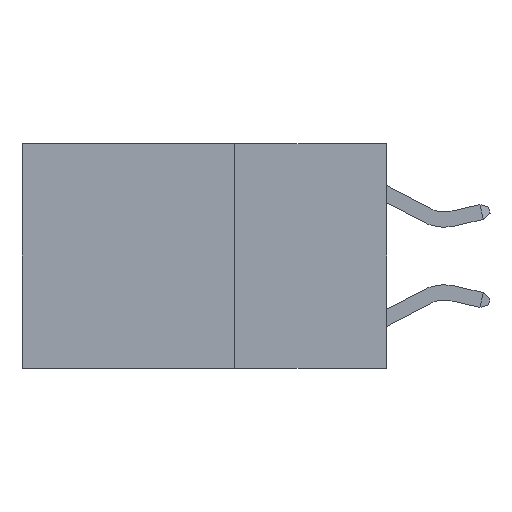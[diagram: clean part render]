
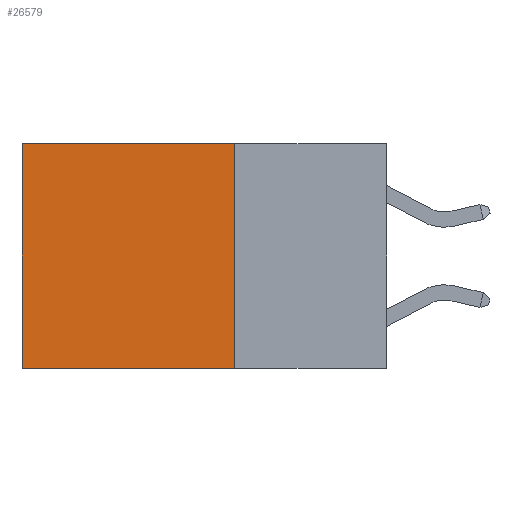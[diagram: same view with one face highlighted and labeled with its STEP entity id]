
A CAD part, left-side view. The second image highlights one B-rep face of the part: STEP entity #26579.
In plain terms, the highlighted planar face has unit normal (-1, 0, 0).
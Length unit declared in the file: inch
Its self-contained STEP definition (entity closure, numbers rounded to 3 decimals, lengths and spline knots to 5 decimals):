
#484 = CARTESIAN_POINT ( 'NONE',  ( 0.2625, 0.6, 0. ) ) ;
#586 = DIRECTION ( 'NONE',  ( 0., 0., -1. ) ) ;
#959 = EDGE_CURVE ( 'NONE', #15453, #30490, #2435, .T. ) ;
#2211 = EDGE_CURVE ( 'NONE', #25527, #30490, #9482, .T. ) ;
#2247 = VECTOR ( 'NONE', #18877, 39.37008 ) ;
#2435 = LINE ( 'NONE', #15923, #2247 ) ;
#2756 = FACE_OUTER_BOUND ( 'NONE', #12522, .T. ) ;
#3754 = CARTESIAN_POINT ( 'NONE',  ( 0.2625, 0.25, 0. ) ) ;
#5227 = CARTESIAN_POINT ( 'NONE',  ( 0.2625, 0.25, 0. ) ) ;
#5386 = ORIENTED_EDGE ( 'NONE', *, *, #21497, .F. ) ;
#6149 = VECTOR ( 'NONE', #12272, 39.37008 ) ;
#6588 = CARTESIAN_POINT ( 'NONE',  ( 0.2625, 0.6, 0. ) ) ;
#6665 = VERTEX_POINT ( 'NONE', #3754 ) ;
#9284 = EDGE_CURVE ( 'NONE', #6665, #25527, #29459, .T. ) ;
#9482 = LINE ( 'NONE', #484, #6149 ) ;
#10420 = VECTOR ( 'NONE', #10786, 39.37008 ) ;
#10786 = DIRECTION ( 'NONE',  ( 0., 1., 0. ) ) ;
#11439 = ORIENTED_EDGE ( 'NONE', *, *, #959, .F. ) ;
#12272 = DIRECTION ( 'NONE',  ( 0., 0., -1. ) ) ;
#12522 = EDGE_LOOP ( 'NONE', ( #25653, #11439, #5386, #27487 ) ) ;
#14356 = CARTESIAN_POINT ( 'NONE',  ( 0.2625, 0.25, 0. ) ) ;
#14821 = LINE ( 'NONE', #14356, #27913 ) ;
#15453 = VERTEX_POINT ( 'NONE', #19519 ) ;
#15923 = CARTESIAN_POINT ( 'NONE',  ( 0.2625, 0.25, -0.37 ) ) ;
#17041 = PLANE ( 'NONE',  #22439 ) ;
#17638 = CARTESIAN_POINT ( 'NONE',  ( 0.2625, 0.25, 0. ) ) ;
#18877 = DIRECTION ( 'NONE',  ( 0., 1., 0. ) ) ;
#19519 = CARTESIAN_POINT ( 'NONE',  ( 0.2625, 0.25, -0.37 ) ) ;
#21497 = EDGE_CURVE ( 'NONE', #6665, #15453, #14821, .T. ) ;
#22439 = AXIS2_PLACEMENT_3D ( 'NONE', #5227, #24196, #586 ) ;
#23253 = DIRECTION ( 'NONE',  ( 0., 0., -1. ) ) ;
#24196 = DIRECTION ( 'NONE',  ( 1., 0., 0. ) ) ;
#25527 = VERTEX_POINT ( 'NONE', #6588 ) ;
#25653 = ORIENTED_EDGE ( 'NONE', *, *, #2211, .T. ) ;
#26579 = ADVANCED_FACE ( 'NONE', ( #2756 ), #17041, .F. ) ;
#27487 = ORIENTED_EDGE ( 'NONE', *, *, #9284, .T. ) ;
#27654 = CARTESIAN_POINT ( 'NONE',  ( 0.2625, 0.6, -0.37 ) ) ;
#27913 = VECTOR ( 'NONE', #23253, 39.37008 ) ;
#29459 = LINE ( 'NONE', #17638, #10420 ) ;
#30490 = VERTEX_POINT ( 'NONE', #27654 ) ;
